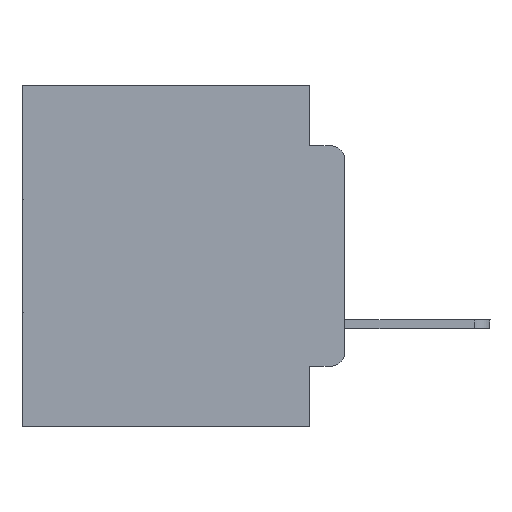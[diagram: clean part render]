
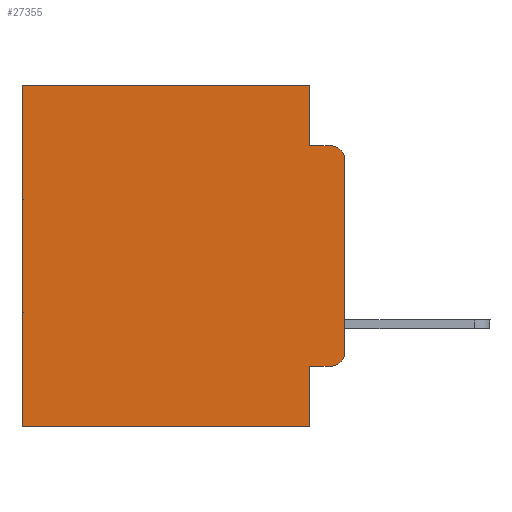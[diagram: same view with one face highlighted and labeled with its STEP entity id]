
A CAD part, left-side view. The second image highlights one B-rep face of the part: STEP entity #27355.
In plain terms, the highlighted planar face has unit normal (-1, 0, 0).
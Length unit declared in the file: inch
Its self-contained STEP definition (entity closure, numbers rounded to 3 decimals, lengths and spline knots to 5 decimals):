
#80 = EDGE_CURVE ( 'NONE', #15340, #17693, #25481, .T. ) ;
#97 = VERTEX_POINT ( 'NONE', #12733 ) ;
#134 = ORIENTED_EDGE ( 'NONE', *, *, #9068, .F. ) ;
#286 = CARTESIAN_POINT ( 'NONE',  ( 0.298, 0.473, -0.5 ) ) ;
#777 = LINE ( 'NONE', #28249, #18078 ) ;
#1503 = EDGE_CURVE ( 'NONE', #14092, #17113, #8603, .T. ) ;
#1579 = DIRECTION ( 'NONE',  ( 0., 0., -1. ) ) ;
#1931 = CARTESIAN_POINT ( 'NONE',  ( 0.298, 0.051, 0. ) ) ;
#1966 = VECTOR ( 'NONE', #11503, 39.37008 ) ;
#2036 = DIRECTION ( 'NONE',  ( 0., 0., -1. ) ) ;
#2288 = CARTESIAN_POINT ( 'NONE',  ( 0.298, 0.473, 0. ) ) ;
#2623 = EDGE_LOOP ( 'NONE', ( #2882, #3987, #17678, #134, #20877, #6821, #8994, #4577, #27593, #20728 ) ) ;
#2882 = ORIENTED_EDGE ( 'NONE', *, *, #7892, .F. ) ;
#3987 = ORIENTED_EDGE ( 'NONE', *, *, #80, .T. ) ;
#4141 = AXIS2_PLACEMENT_3D ( 'NONE', #28630, #13089, #2036 ) ;
#4261 = LINE ( 'NONE', #28342, #22171 ) ;
#4271 = DIRECTION ( 'NONE',  ( 0., 0., -1. ) ) ;
#4577 = ORIENTED_EDGE ( 'NONE', *, *, #5676, .F. ) ;
#4699 = CARTESIAN_POINT ( 'NONE',  ( 0.298, 0.051, 0. ) ) ;
#4836 = PLANE ( 'NONE',  #14197 ) ;
#5676 = EDGE_CURVE ( 'NONE', #13323, #19168, #7966, .T. ) ;
#6047 = EDGE_CURVE ( 'NONE', #19168, #19653, #27575, .T. ) ;
#6147 = VECTOR ( 'NONE', #14190, 39.37008 ) ;
#6821 = ORIENTED_EDGE ( 'NONE', *, *, #17645, .T. ) ;
#7173 = CARTESIAN_POINT ( 'NONE',  ( 0.298, 0., 0. ) ) ;
#7892 = EDGE_CURVE ( 'NONE', #15340, #97, #777, .T. ) ;
#7966 = LINE ( 'NONE', #4699, #1966 ) ;
#8232 = LINE ( 'NONE', #26911, #17062 ) ;
#8281 = CARTESIAN_POINT ( 'NONE',  ( 0.298, 0.051, -0.4115 ) ) ;
#8469 = CARTESIAN_POINT ( 'NONE',  ( 0.298, 0., -0.1085 ) ) ;
#8603 = LINE ( 'NONE', #7173, #6147 ) ;
#8994 = ORIENTED_EDGE ( 'NONE', *, *, #6047, .F. ) ;
#9068 = EDGE_CURVE ( 'NONE', #14092, #23148, #4261, .T. ) ;
#9386 = FACE_OUTER_BOUND ( 'NONE', #2623, .T. ) ;
#11503 = DIRECTION ( 'NONE',  ( 0., 0., -1. ) ) ;
#11636 = DIRECTION ( 'NONE',  ( 1., 0., 0. ) ) ;
#12655 = VECTOR ( 'NONE', #4271, 39.37008 ) ;
#12733 = CARTESIAN_POINT ( 'NONE',  ( 0.298, 0., -0.3915 ) ) ;
#13089 = DIRECTION ( 'NONE',  ( -1., 0., 0. ) ) ;
#13323 = VERTEX_POINT ( 'NONE', #8281 ) ;
#13720 = CARTESIAN_POINT ( 'NONE',  ( 0.298, 0.051, -0.0885 ) ) ;
#13954 = CARTESIAN_POINT ( 'NONE',  ( 0.298, 0.051, -0.5 ) ) ;
#14080 = EDGE_CURVE ( 'NONE', #21126, #97, #20069, .T. ) ;
#14092 = VERTEX_POINT ( 'NONE', #1931 ) ;
#14190 = DIRECTION ( 'NONE',  ( 0., 1., 0. ) ) ;
#14197 = AXIS2_PLACEMENT_3D ( 'NONE', #25044, #11636, #27290 ) ;
#14770 = CARTESIAN_POINT ( 'NONE',  ( 0.298, 0., -0.5 ) ) ;
#15340 = VERTEX_POINT ( 'NONE', #8469 ) ;
#15502 = LINE ( 'NONE', #2288, #12655 ) ;
#17037 = DIRECTION ( 'NONE',  ( 0., 0., -1. ) ) ;
#17062 = VECTOR ( 'NONE', #22210, 39.37008 ) ;
#17113 = VERTEX_POINT ( 'NONE', #21611 ) ;
#17316 = DIRECTION ( 'NONE',  ( 0., 0., -1. ) ) ;
#17645 = EDGE_CURVE ( 'NONE', #17113, #19653, #15502, .T. ) ;
#17678 = ORIENTED_EDGE ( 'NONE', *, *, #23287, .F. ) ;
#17693 = VERTEX_POINT ( 'NONE', #26722 ) ;
#18078 = VECTOR ( 'NONE', #17037, 39.37008 ) ;
#19168 = VERTEX_POINT ( 'NONE', #13954 ) ;
#19332 = DIRECTION ( 'NONE',  ( 0., 1., 0. ) ) ;
#19540 = VECTOR ( 'NONE', #19332, 39.37008 ) ;
#19653 = VERTEX_POINT ( 'NONE', #286 ) ;
#20069 = CIRCLE ( 'NONE', #4141, 0.02 ) ;
#20245 = AXIS2_PLACEMENT_3D ( 'NONE', #26126, #28471, #1579 ) ;
#20382 = DIRECTION ( 'NONE',  ( 0., -1., 0. ) ) ;
#20728 = ORIENTED_EDGE ( 'NONE', *, *, #14080, .T. ) ;
#20877 = ORIENTED_EDGE ( 'NONE', *, *, #1503, .T. ) ;
#21126 = VERTEX_POINT ( 'NONE', #28054 ) ;
#21225 = LINE ( 'NONE', #13720, #26123 ) ;
#21301 = CARTESIAN_POINT ( 'NONE',  ( 0.298, 0.051, -0.0885 ) ) ;
#21611 = CARTESIAN_POINT ( 'NONE',  ( 0.298, 0.473, 0. ) ) ;
#22171 = VECTOR ( 'NONE', #17316, 39.37008 ) ;
#22210 = DIRECTION ( 'NONE',  ( 0., -1., 0. ) ) ;
#22644 = EDGE_CURVE ( 'NONE', #13323, #21126, #8232, .T. ) ;
#23148 = VERTEX_POINT ( 'NONE', #21301 ) ;
#23287 = EDGE_CURVE ( 'NONE', #23148, #17693, #21225, .T. ) ;
#25044 = CARTESIAN_POINT ( 'NONE',  ( 0.298, 0., 0. ) ) ;
#25481 = CIRCLE ( 'NONE', #20245, 0.02 ) ;
#26123 = VECTOR ( 'NONE', #20382, 39.37008 ) ;
#26126 = CARTESIAN_POINT ( 'NONE',  ( 0.298, 0.02, -0.1085 ) ) ;
#26722 = CARTESIAN_POINT ( 'NONE',  ( 0.298, 0.02, -0.0885 ) ) ;
#26911 = CARTESIAN_POINT ( 'NONE',  ( 0.298, 0.051, -0.4115 ) ) ;
#27290 = DIRECTION ( 'NONE',  ( 0., 0., -1. ) ) ;
#27355 = ADVANCED_FACE ( 'NONE', ( #9386 ), #4836, .F. ) ;
#27575 = LINE ( 'NONE', #14770, #19540 ) ;
#27593 = ORIENTED_EDGE ( 'NONE', *, *, #22644, .T. ) ;
#28054 = CARTESIAN_POINT ( 'NONE',  ( 0.298, 0.02, -0.4115 ) ) ;
#28249 = CARTESIAN_POINT ( 'NONE',  ( 0.298, 0., 0. ) ) ;
#28342 = CARTESIAN_POINT ( 'NONE',  ( 0.298, 0.051, 0. ) ) ;
#28471 = DIRECTION ( 'NONE',  ( -1., 0., 0. ) ) ;
#28630 = CARTESIAN_POINT ( 'NONE',  ( 0.298, 0.02, -0.3915 ) ) ;
